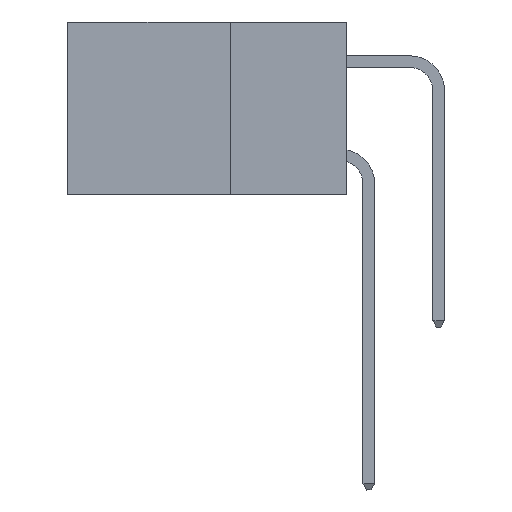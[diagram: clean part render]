
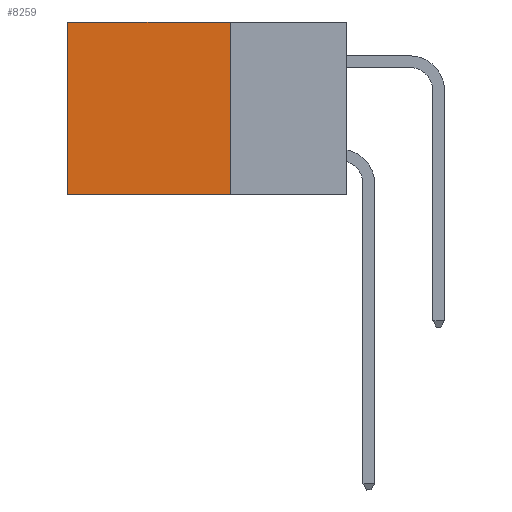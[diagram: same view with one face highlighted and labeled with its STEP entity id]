
A CAD part, left-side view. The second image highlights one B-rep face of the part: STEP entity #8259.
In plain terms, the highlighted planar face has unit normal (-1, 0, 0).
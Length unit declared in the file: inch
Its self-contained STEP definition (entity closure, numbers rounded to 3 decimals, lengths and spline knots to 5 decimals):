
#55 = LINE ( 'NONE', #199, #16886 ) ;
#167 = VECTOR ( 'NONE', #10166, 39.37008 ) ;
#199 = CARTESIAN_POINT ( 'NONE',  ( 0.2875, 0.25, 0. ) ) ;
#808 = CARTESIAN_POINT ( 'NONE',  ( 0.2875, 0.6, 0. ) ) ;
#2108 = VERTEX_POINT ( 'NONE', #19705 ) ;
#2895 = DIRECTION ( 'NONE',  ( 0., 0., -1. ) ) ;
#3431 = VERTEX_POINT ( 'NONE', #20148 ) ;
#4715 = VECTOR ( 'NONE', #28528, 39.37008 ) ;
#5428 = CARTESIAN_POINT ( 'NONE',  ( 0.2875, 0.25, -0.37 ) ) ;
#6362 = EDGE_CURVE ( 'NONE', #29059, #11792, #21775, .T. ) ;
#7711 = VECTOR ( 'NONE', #2895, 39.37008 ) ;
#8259 = ADVANCED_FACE ( 'NONE', ( #19696 ), #10548, .F. ) ;
#8341 = DIRECTION ( 'NONE',  ( 0., 0., -1. ) ) ;
#8484 = DIRECTION ( 'NONE',  ( 1., 0., 0. ) ) ;
#10166 = DIRECTION ( 'NONE',  ( 0., 1., 0. ) ) ;
#10548 = PLANE ( 'NONE',  #11843 ) ;
#11398 = EDGE_CURVE ( 'NONE', #3431, #11792, #19159, .T. ) ;
#11792 = VERTEX_POINT ( 'NONE', #19418 ) ;
#11843 = AXIS2_PLACEMENT_3D ( 'NONE', #12467, #8484, #8341 ) ;
#12467 = CARTESIAN_POINT ( 'NONE',  ( 0.2875, 0.25, 0. ) ) ;
#14993 = CARTESIAN_POINT ( 'NONE',  ( 0.2875, 0.6, 0. ) ) ;
#15663 = ORIENTED_EDGE ( 'NONE', *, *, #11398, .F. ) ;
#16886 = VECTOR ( 'NONE', #20004, 39.37008 ) ;
#19159 = LINE ( 'NONE', #5428, #167 ) ;
#19418 = CARTESIAN_POINT ( 'NONE',  ( 0.2875, 0.6, -0.37 ) ) ;
#19500 = LINE ( 'NONE', #21434, #4715 ) ;
#19696 = FACE_OUTER_BOUND ( 'NONE', #28396, .T. ) ;
#19705 = CARTESIAN_POINT ( 'NONE',  ( 0.2875, 0.25, 0. ) ) ;
#20004 = DIRECTION ( 'NONE',  ( 0., 1., 0. ) ) ;
#20148 = CARTESIAN_POINT ( 'NONE',  ( 0.2875, 0.25, -0.37 ) ) ;
#20886 = EDGE_CURVE ( 'NONE', #2108, #29059, #55, .T. ) ;
#21224 = ORIENTED_EDGE ( 'NONE', *, *, #20886, .T. ) ;
#21434 = CARTESIAN_POINT ( 'NONE',  ( 0.2875, 0.25, 0. ) ) ;
#21775 = LINE ( 'NONE', #808, #7711 ) ;
#21890 = ORIENTED_EDGE ( 'NONE', *, *, #22784, .F. ) ;
#22784 = EDGE_CURVE ( 'NONE', #2108, #3431, #19500, .T. ) ;
#27285 = ORIENTED_EDGE ( 'NONE', *, *, #6362, .T. ) ;
#28396 = EDGE_LOOP ( 'NONE', ( #27285, #15663, #21890, #21224 ) ) ;
#28528 = DIRECTION ( 'NONE',  ( 0., 0., -1. ) ) ;
#29059 = VERTEX_POINT ( 'NONE', #14993 ) ;
